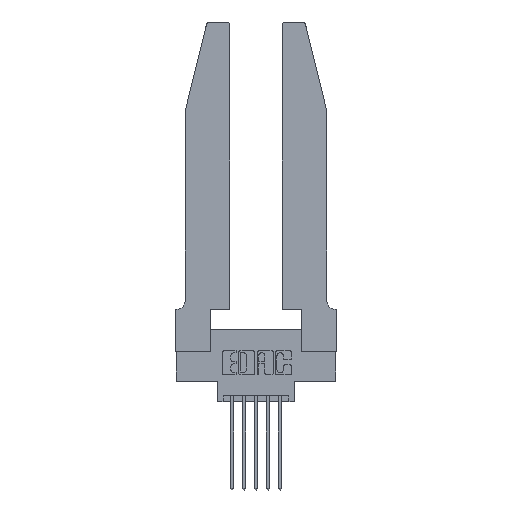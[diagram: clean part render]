
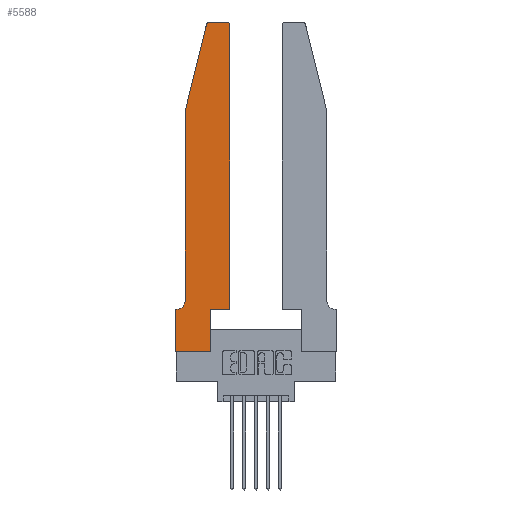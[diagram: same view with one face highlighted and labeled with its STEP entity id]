
A CAD part, top view. The second image highlights one B-rep face of the part: STEP entity #5588.
In plain terms, the highlighted planar face has unit normal (0, 0, 1).
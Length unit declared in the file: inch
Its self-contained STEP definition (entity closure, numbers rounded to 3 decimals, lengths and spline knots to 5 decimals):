
#76 = DIRECTION ( 'NONE',  ( 1., 0., 0. ) ) ;
#92 = CARTESIAN_POINT ( 'NONE',  ( 0.4205, 2.75, 0.37 ) ) ;
#255 = VERTEX_POINT ( 'NONE', #10933 ) ;
#332 = ORIENTED_EDGE ( 'NONE', *, *, #11848, .T. ) ;
#344 = EDGE_LOOP ( 'NONE', ( #3835, #13738, #332, #12249, #6672, #2258, #1061, #11199, #13381, #690, #7994, #11648 ) ) ;
#476 = VERTEX_POINT ( 'NONE', #2702 ) ;
#545 = VECTOR ( 'NONE', #8057, 39.37008 ) ;
#690 = ORIENTED_EDGE ( 'NONE', *, *, #10129, .T. ) ;
#982 = VECTOR ( 'NONE', #1800, 39.37008 ) ;
#1010 = VERTEX_POINT ( 'NONE', #92 ) ;
#1061 = ORIENTED_EDGE ( 'NONE', *, *, #2362, .T. ) ;
#1117 = VECTOR ( 'NONE', #12257, 39.37008 ) ;
#1149 = EDGE_CURVE ( 'NONE', #3116, #7356, #6837, .T. ) ;
#1179 = CARTESIAN_POINT ( 'NONE',  ( 0.2865, 0., 0.37 ) ) ;
#1777 = CARTESIAN_POINT ( 'NONE',  ( 0.4205, 2.72, 0.37 ) ) ;
#1800 = DIRECTION ( 'NONE',  ( 0., 1., 0. ) ) ;
#1814 = CARTESIAN_POINT ( 'NONE',  ( 0.4505, 0.35, 0.37 ) ) ;
#1995 = VERTEX_POINT ( 'NONE', #7453 ) ;
#2184 = EDGE_CURVE ( 'NONE', #1995, #476, #9555, .T. ) ;
#2258 = ORIENTED_EDGE ( 'NONE', *, *, #5505, .T. ) ;
#2362 = EDGE_CURVE ( 'NONE', #5404, #7789, #4821, .T. ) ;
#2491 = LINE ( 'NONE', #7525, #10654 ) ;
#2550 = VECTOR ( 'NONE', #76, 39.37008 ) ;
#2640 = CARTESIAN_POINT ( 'NONE',  ( 0., 0.35, 0.37 ) ) ;
#2702 = CARTESIAN_POINT ( 'NONE',  ( 0.0755, 0.42, 0.37 ) ) ;
#2765 = DIRECTION ( 'NONE',  ( 0., -1., 0. ) ) ;
#2901 = DIRECTION ( 'NONE',  ( 1., 0., 0. ) ) ;
#3116 = VERTEX_POINT ( 'NONE', #3433 ) ;
#3433 = CARTESIAN_POINT ( 'NONE',  ( 0.4505, 0.35, 0.37 ) ) ;
#3631 = AXIS2_PLACEMENT_3D ( 'NONE', #5008, #12283, #6082 ) ;
#3633 = CIRCLE ( 'NONE', #3631, 0.07 ) ;
#3770 = VECTOR ( 'NONE', #10632, 39.37008 ) ;
#3835 = ORIENTED_EDGE ( 'NONE', *, *, #11457, .T. ) ;
#3864 = LINE ( 'NONE', #4702, #6404 ) ;
#3865 = CARTESIAN_POINT ( 'NONE',  ( 0.0755, 2., 0.37 ) ) ;
#3874 = CARTESIAN_POINT ( 'NONE',  ( 0.4505, 2.72, 0.37 ) ) ;
#4555 = CARTESIAN_POINT ( 'NONE',  ( 0., 0., 0.37 ) ) ;
#4589 = CARTESIAN_POINT ( 'NONE',  ( 0., 0.35, 0.37 ) ) ;
#4702 = CARTESIAN_POINT ( 'NONE',  ( 0.0755, 0.35, 0.37 ) ) ;
#4821 = LINE ( 'NONE', #5904, #10043 ) ;
#4893 = PLANE ( 'NONE',  #12447 ) ;
#5008 = CARTESIAN_POINT ( 'NONE',  ( 0.0055, 0.42, 0.37 ) ) ;
#5404 = VERTEX_POINT ( 'NONE', #4589 ) ;
#5495 = LINE ( 'NONE', #4555, #2550 ) ;
#5505 = EDGE_CURVE ( 'NONE', #11075, #5404, #3864, .T. ) ;
#5528 = AXIS2_PLACEMENT_3D ( 'NONE', #12565, #6369, #13572 ) ;
#5531 = VERTEX_POINT ( 'NONE', #7934 ) ;
#5588 = ADVANCED_FACE ( 'NONE', ( #5743 ), #4893, .T. ) ;
#5629 = CARTESIAN_POINT ( 'NONE',  ( 0.2865, 0.35, 0.37 ) ) ;
#5743 = FACE_OUTER_BOUND ( 'NONE', #344, .T. ) ;
#5801 = DIRECTION ( 'NONE',  ( 0., -1., 0. ) ) ;
#5904 = CARTESIAN_POINT ( 'NONE',  ( 0., 0., 0.37 ) ) ;
#5966 = DIRECTION ( 'NONE',  ( 1., 0., 0. ) ) ;
#6056 = VERTEX_POINT ( 'NONE', #5629 ) ;
#6082 = DIRECTION ( 'NONE',  ( -1., 0., 0. ) ) ;
#6369 = DIRECTION ( 'NONE',  ( 0., 0., 1. ) ) ;
#6404 = VECTOR ( 'NONE', #8928, 39.37008 ) ;
#6649 = LINE ( 'NONE', #8550, #3770 ) ;
#6672 = ORIENTED_EDGE ( 'NONE', *, *, #6724, .T. ) ;
#6724 = EDGE_CURVE ( 'NONE', #476, #11075, #3633, .T. ) ;
#6837 = LINE ( 'NONE', #1814, #982 ) ;
#6894 = CARTESIAN_POINT ( 'NONE',  ( 0.0055, 0.35, 0.37 ) ) ;
#7356 = VERTEX_POINT ( 'NONE', #3874 ) ;
#7453 = CARTESIAN_POINT ( 'NONE',  ( 0.0755, 2., 0.37 ) ) ;
#7525 = CARTESIAN_POINT ( 'NONE',  ( 0.2605, 2.75, 0.37 ) ) ;
#7789 = VERTEX_POINT ( 'NONE', #11749 ) ;
#7934 = CARTESIAN_POINT ( 'NONE',  ( 0.25487, 2.72718, 0.37 ) ) ;
#7994 = ORIENTED_EDGE ( 'NONE', *, *, #1149, .T. ) ;
#8057 = DIRECTION ( 'NONE',  ( -0.239, -0.971, 0. ) ) ;
#8165 = CARTESIAN_POINT ( 'NONE',  ( 0.0755, 2., 0.37 ) ) ;
#8417 = CIRCLE ( 'NONE', #5528, 0.03 ) ;
#8550 = CARTESIAN_POINT ( 'NONE',  ( 0.2865, 0.35, 0.37 ) ) ;
#8928 = DIRECTION ( 'NONE',  ( -1., 0., 0. ) ) ;
#9181 = LINE ( 'NONE', #3865, #545 ) ;
#9237 = VECTOR ( 'NONE', #2765, 39.37008 ) ;
#9296 = DIRECTION ( 'NONE',  ( 0., 0., 1. ) ) ;
#9467 = AXIS2_PLACEMENT_3D ( 'NONE', #1777, #9296, #2901 ) ;
#9488 = EDGE_CURVE ( 'NONE', #7789, #13726, #5495, .T. ) ;
#9555 = LINE ( 'NONE', #8165, #9237 ) ;
#10043 = VECTOR ( 'NONE', #5801, 39.37008 ) ;
#10129 = EDGE_CURVE ( 'NONE', #6056, #3116, #12463, .T. ) ;
#10175 = CARTESIAN_POINT ( 'NONE',  ( 0.4505, 0.35, 0.37 ) ) ;
#10272 = EDGE_CURVE ( 'NONE', #255, #5531, #8417, .T. ) ;
#10632 = DIRECTION ( 'NONE',  ( 0., 1., 0. ) ) ;
#10647 = DIRECTION ( 'NONE',  ( -1., 0., 0. ) ) ;
#10654 = VECTOR ( 'NONE', #10647, 39.37008 ) ;
#10705 = CIRCLE ( 'NONE', #9467, 0.03 ) ;
#10933 = CARTESIAN_POINT ( 'NONE',  ( 0.284, 2.75, 0.37 ) ) ;
#11075 = VERTEX_POINT ( 'NONE', #6894 ) ;
#11199 = ORIENTED_EDGE ( 'NONE', *, *, #9488, .T. ) ;
#11457 = EDGE_CURVE ( 'NONE', #1010, #255, #2491, .T. ) ;
#11648 = ORIENTED_EDGE ( 'NONE', *, *, #12454, .T. ) ;
#11749 = CARTESIAN_POINT ( 'NONE',  ( 0., 0., 0.37 ) ) ;
#11848 = EDGE_CURVE ( 'NONE', #5531, #1995, #9181, .T. ) ;
#12096 = EDGE_CURVE ( 'NONE', #13726, #6056, #6649, .T. ) ;
#12170 = DIRECTION ( 'NONE',  ( 0., 0., 1. ) ) ;
#12249 = ORIENTED_EDGE ( 'NONE', *, *, #2184, .T. ) ;
#12257 = DIRECTION ( 'NONE',  ( 1., 0., 0. ) ) ;
#12283 = DIRECTION ( 'NONE',  ( 0., 0., -1. ) ) ;
#12447 = AXIS2_PLACEMENT_3D ( 'NONE', #2640, #12170, #5966 ) ;
#12454 = EDGE_CURVE ( 'NONE', #7356, #1010, #10705, .T. ) ;
#12463 = LINE ( 'NONE', #10175, #1117 ) ;
#12565 = CARTESIAN_POINT ( 'NONE',  ( 0.284, 2.72, 0.37 ) ) ;
#13381 = ORIENTED_EDGE ( 'NONE', *, *, #12096, .T. ) ;
#13572 = DIRECTION ( 'NONE',  ( 1., 0., 0. ) ) ;
#13726 = VERTEX_POINT ( 'NONE', #1179 ) ;
#13738 = ORIENTED_EDGE ( 'NONE', *, *, #10272, .T. ) ;
